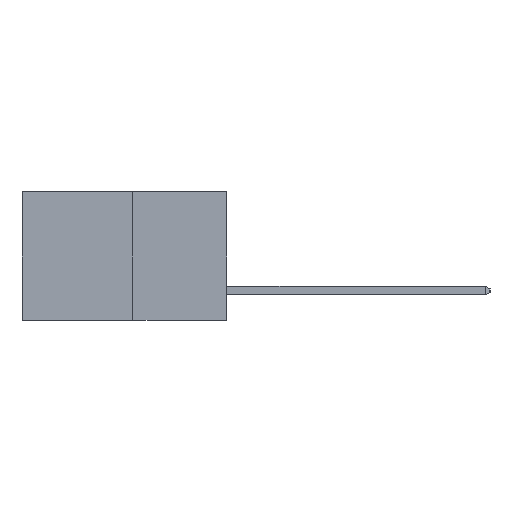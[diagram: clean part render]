
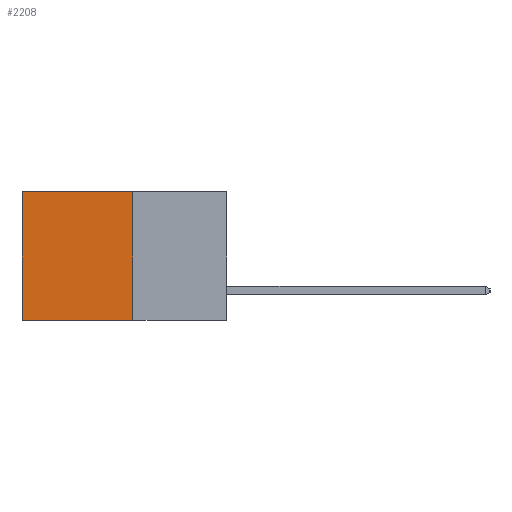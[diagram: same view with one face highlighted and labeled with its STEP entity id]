
A CAD part, left-side view. The second image highlights one B-rep face of the part: STEP entity #2208.
In plain terms, the highlighted planar face has unit normal (-1, 0, 0).
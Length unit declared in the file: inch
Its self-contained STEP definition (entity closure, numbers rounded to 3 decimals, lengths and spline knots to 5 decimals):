
#8 = VECTOR ( 'NONE', #16792, 39.37008 ) ;
#734 = LINE ( 'NONE', #1387, #8 ) ;
#1387 = CARTESIAN_POINT ( 'NONE',  ( 0.277, 0.27, -0.37 ) ) ;
#2208 = ADVANCED_FACE ( 'NONE', ( #9484 ), #14763, .F. ) ;
#2230 = CARTESIAN_POINT ( 'NONE',  ( 0.277, 0.59, -0.37 ) ) ;
#3873 = EDGE_CURVE ( 'NONE', #22509, #23550, #26639, .T. ) ;
#9484 = FACE_OUTER_BOUND ( 'NONE', #12975, .T. ) ;
#10228 = CARTESIAN_POINT ( 'NONE',  ( 0.277, 0.27, 0. ) ) ;
#12910 = CARTESIAN_POINT ( 'NONE',  ( 0.277, 0.27, -0.37 ) ) ;
#12975 = EDGE_LOOP ( 'NONE', ( #16498, #21643, #20234, #16017 ) ) ;
#14763 = PLANE ( 'NONE',  #19051 ) ;
#14784 = VERTEX_POINT ( 'NONE', #19324 ) ;
#14933 = VERTEX_POINT ( 'NONE', #17619 ) ;
#15065 = DIRECTION ( 'NONE',  ( 0., 0., -1. ) ) ;
#15105 = VECTOR ( 'NONE', #20259, 39.37008 ) ;
#16017 = ORIENTED_EDGE ( 'NONE', *, *, #21675, .T. ) ;
#16080 = CARTESIAN_POINT ( 'NONE',  ( 0.277, 0.27, -0.37 ) ) ;
#16175 = LINE ( 'NONE', #10228, #16857 ) ;
#16277 = DIRECTION ( 'NONE',  ( 0., 0., -1. ) ) ;
#16368 = DIRECTION ( 'NONE',  ( 1., 0., 0. ) ) ;
#16498 = ORIENTED_EDGE ( 'NONE', *, *, #3873, .T. ) ;
#16792 = DIRECTION ( 'NONE',  ( 0., 1., 0. ) ) ;
#16857 = VECTOR ( 'NONE', #25375, 39.37008 ) ;
#17619 = CARTESIAN_POINT ( 'NONE',  ( 0.277, 0.27, -0.37 ) ) ;
#19051 = AXIS2_PLACEMENT_3D ( 'NONE', #16080, #16368, #16277 ) ;
#19324 = CARTESIAN_POINT ( 'NONE',  ( 0.277, 0.27, 0. ) ) ;
#19451 = EDGE_CURVE ( 'NONE', #14784, #14933, #25308, .T. ) ;
#20234 = ORIENTED_EDGE ( 'NONE', *, *, #19451, .F. ) ;
#20259 = DIRECTION ( 'NONE',  ( 0., 0., -1. ) ) ;
#20359 = CARTESIAN_POINT ( 'NONE',  ( 0.277, 0.59, -0.37 ) ) ;
#21620 = CARTESIAN_POINT ( 'NONE',  ( 0.277, 0.59, 0. ) ) ;
#21643 = ORIENTED_EDGE ( 'NONE', *, *, #25133, .F. ) ;
#21675 = EDGE_CURVE ( 'NONE', #14784, #22509, #16175, .T. ) ;
#22509 = VERTEX_POINT ( 'NONE', #21620 ) ;
#23550 = VERTEX_POINT ( 'NONE', #2230 ) ;
#23949 = VECTOR ( 'NONE', #15065, 39.37008 ) ;
#25133 = EDGE_CURVE ( 'NONE', #14933, #23550, #734, .T. ) ;
#25308 = LINE ( 'NONE', #12910, #23949 ) ;
#25375 = DIRECTION ( 'NONE',  ( 0., 1., 0. ) ) ;
#26639 = LINE ( 'NONE', #20359, #15105 ) ;
